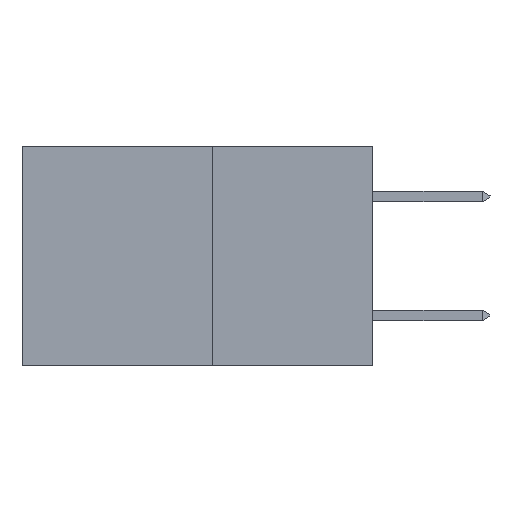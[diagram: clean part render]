
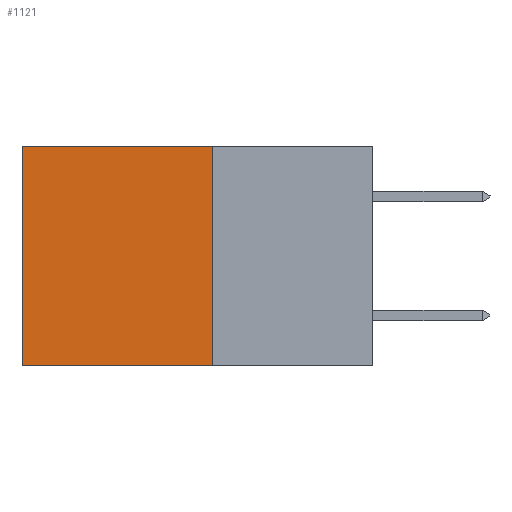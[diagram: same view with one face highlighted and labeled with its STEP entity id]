
A CAD part, left-side view. The second image highlights one B-rep face of the part: STEP entity #1121.
In plain terms, the highlighted planar face has unit normal (-1, 0, 0).
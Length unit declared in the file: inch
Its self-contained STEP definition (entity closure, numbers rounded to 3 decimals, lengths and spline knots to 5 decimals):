
#420 = ORIENTED_EDGE ( 'NONE', *, *, #4415, .T. ) ;
#758 = ORIENTED_EDGE ( 'NONE', *, *, #2550, .F. ) ;
#810 = CARTESIAN_POINT ( 'NONE',  ( 0.277, 0.27, -0.37 ) ) ;
#1066 = VECTOR ( 'NONE', #5530, 39.37008 ) ;
#1121 = ADVANCED_FACE ( 'NONE', ( #8450 ), #7691, .F. ) ;
#1311 = EDGE_CURVE ( 'NONE', #5870, #3141, #7762, .T. ) ;
#1370 = VERTEX_POINT ( 'NONE', #2936 ) ;
#2091 = DIRECTION ( 'NONE',  ( 0., 0., -1. ) ) ;
#2550 = EDGE_CURVE ( 'NONE', #5870, #1370, #6474, .T. ) ;
#2684 = EDGE_LOOP ( 'NONE', ( #420, #7018, #758, #4203 ) ) ;
#2833 = DIRECTION ( 'NONE',  ( 0., 1., 0. ) ) ;
#2928 = CARTESIAN_POINT ( 'NONE',  ( 0.277, 0.59, -0.37 ) ) ;
#2936 = CARTESIAN_POINT ( 'NONE',  ( 0.277, 0.27, -0.37 ) ) ;
#3141 = VERTEX_POINT ( 'NONE', #3399 ) ;
#3341 = DIRECTION ( 'NONE',  ( 1., 0., 0. ) ) ;
#3365 = LINE ( 'NONE', #8738, #1066 ) ;
#3399 = CARTESIAN_POINT ( 'NONE',  ( 0.277, 0.59, 0. ) ) ;
#4203 = ORIENTED_EDGE ( 'NONE', *, *, #1311, .T. ) ;
#4357 = CARTESIAN_POINT ( 'NONE',  ( 0.277, 0.59, -0.37 ) ) ;
#4415 = EDGE_CURVE ( 'NONE', #3141, #7585, #5720, .T. ) ;
#5530 = DIRECTION ( 'NONE',  ( 0., 1., 0. ) ) ;
#5720 = LINE ( 'NONE', #2928, #6154 ) ;
#5870 = VERTEX_POINT ( 'NONE', #8392 ) ;
#6154 = VECTOR ( 'NONE', #7734, 39.37008 ) ;
#6228 = AXIS2_PLACEMENT_3D ( 'NONE', #810, #3341, #2091 ) ;
#6474 = LINE ( 'NONE', #8371, #6686 ) ;
#6686 = VECTOR ( 'NONE', #8671, 39.37008 ) ;
#7018 = ORIENTED_EDGE ( 'NONE', *, *, #8494, .F. ) ;
#7575 = VECTOR ( 'NONE', #2833, 39.37008 ) ;
#7585 = VERTEX_POINT ( 'NONE', #4357 ) ;
#7691 = PLANE ( 'NONE',  #6228 ) ;
#7734 = DIRECTION ( 'NONE',  ( 0., 0., -1. ) ) ;
#7762 = LINE ( 'NONE', #8702, #7575 ) ;
#8371 = CARTESIAN_POINT ( 'NONE',  ( 0.277, 0.27, -0.37 ) ) ;
#8392 = CARTESIAN_POINT ( 'NONE',  ( 0.277, 0.27, 0. ) ) ;
#8450 = FACE_OUTER_BOUND ( 'NONE', #2684, .T. ) ;
#8494 = EDGE_CURVE ( 'NONE', #1370, #7585, #3365, .T. ) ;
#8671 = DIRECTION ( 'NONE',  ( 0., 0., -1. ) ) ;
#8702 = CARTESIAN_POINT ( 'NONE',  ( 0.277, 0.27, 0. ) ) ;
#8738 = CARTESIAN_POINT ( 'NONE',  ( 0.277, 0.27, -0.37 ) ) ;
